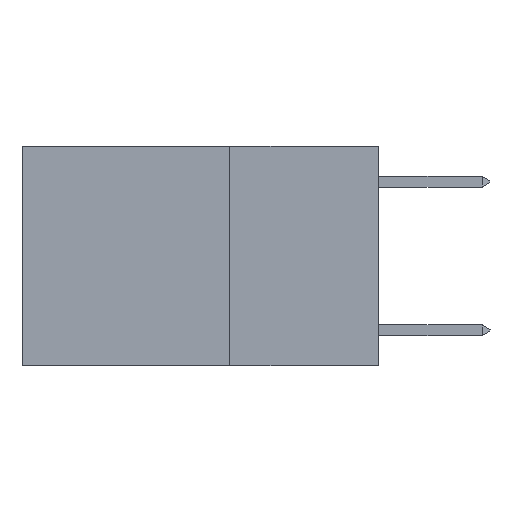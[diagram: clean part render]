
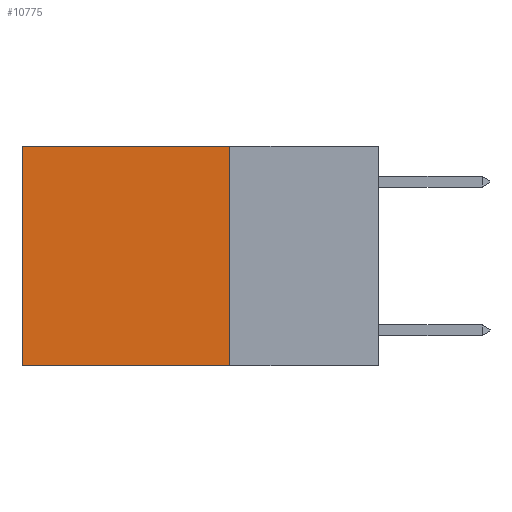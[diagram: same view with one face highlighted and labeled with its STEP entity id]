
A CAD part, left-side view. The second image highlights one B-rep face of the part: STEP entity #10775.
In plain terms, the highlighted planar face has unit normal (-1, 0, 0).
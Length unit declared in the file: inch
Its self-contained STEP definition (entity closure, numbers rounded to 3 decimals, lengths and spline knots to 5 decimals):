
#468 = FACE_OUTER_BOUND ( 'NONE', #11394, .T. ) ;
#2265 = AXIS2_PLACEMENT_3D ( 'NONE', #7681, #4818, #17242 ) ;
#2415 = LINE ( 'NONE', #12717, #7604 ) ;
#3056 = LINE ( 'NONE', #14868, #14248 ) ;
#3118 = ORIENTED_EDGE ( 'NONE', *, *, #5132, .T. ) ;
#3373 = CARTESIAN_POINT ( 'NONE',  ( 0.2625, 0.6, -0.37 ) ) ;
#4818 = DIRECTION ( 'NONE',  ( 1., 0., 0. ) ) ;
#5132 = EDGE_CURVE ( 'NONE', #17030, #17502, #16543, .T. ) ;
#7278 = VECTOR ( 'NONE', #11074, 39.37008 ) ;
#7532 = ORIENTED_EDGE ( 'NONE', *, *, #8144, .T. ) ;
#7604 = VECTOR ( 'NONE', #14037, 39.37008 ) ;
#7681 = CARTESIAN_POINT ( 'NONE',  ( 0.2625, 0.25, 0. ) ) ;
#8064 = DIRECTION ( 'NONE',  ( 0., 1., 0. ) ) ;
#8144 = EDGE_CURVE ( 'NONE', #17502, #10560, #2415, .T. ) ;
#9245 = PLANE ( 'NONE',  #2265 ) ;
#9785 = DIRECTION ( 'NONE',  ( 0., 0., -1. ) ) ;
#10007 = CARTESIAN_POINT ( 'NONE',  ( 0.2625, 0.25, -0.37 ) ) ;
#10560 = VERTEX_POINT ( 'NONE', #3373 ) ;
#10775 = ADVANCED_FACE ( 'NONE', ( #468 ), #9245, .F. ) ;
#11074 = DIRECTION ( 'NONE',  ( 0., 1., 0. ) ) ;
#11345 = ORIENTED_EDGE ( 'NONE', *, *, #12594, .F. ) ;
#11394 = EDGE_LOOP ( 'NONE', ( #7532, #13070, #11345, #3118 ) ) ;
#12039 = EDGE_CURVE ( 'NONE', #12772, #10560, #3056, .T. ) ;
#12416 = CARTESIAN_POINT ( 'NONE',  ( 0.2625, 0.6, 0. ) ) ;
#12594 = EDGE_CURVE ( 'NONE', #17030, #12772, #14451, .T. ) ;
#12717 = CARTESIAN_POINT ( 'NONE',  ( 0.2625, 0.6, 0. ) ) ;
#12772 = VERTEX_POINT ( 'NONE', #10007 ) ;
#13070 = ORIENTED_EDGE ( 'NONE', *, *, #12039, .F. ) ;
#14037 = DIRECTION ( 'NONE',  ( 0., 0., -1. ) ) ;
#14248 = VECTOR ( 'NONE', #8064, 39.37008 ) ;
#14451 = LINE ( 'NONE', #15140, #17655 ) ;
#14868 = CARTESIAN_POINT ( 'NONE',  ( 0.2625, 0.25, -0.37 ) ) ;
#15140 = CARTESIAN_POINT ( 'NONE',  ( 0.2625, 0.25, 0. ) ) ;
#15508 = CARTESIAN_POINT ( 'NONE',  ( 0.2625, 0.25, 0. ) ) ;
#16543 = LINE ( 'NONE', #17737, #7278 ) ;
#17030 = VERTEX_POINT ( 'NONE', #15508 ) ;
#17242 = DIRECTION ( 'NONE',  ( 0., 0., -1. ) ) ;
#17502 = VERTEX_POINT ( 'NONE', #12416 ) ;
#17655 = VECTOR ( 'NONE', #9785, 39.37008 ) ;
#17737 = CARTESIAN_POINT ( 'NONE',  ( 0.2625, 0.25, 0. ) ) ;
